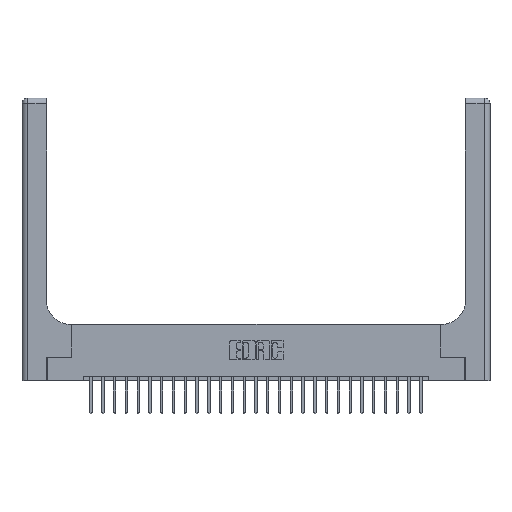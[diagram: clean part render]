
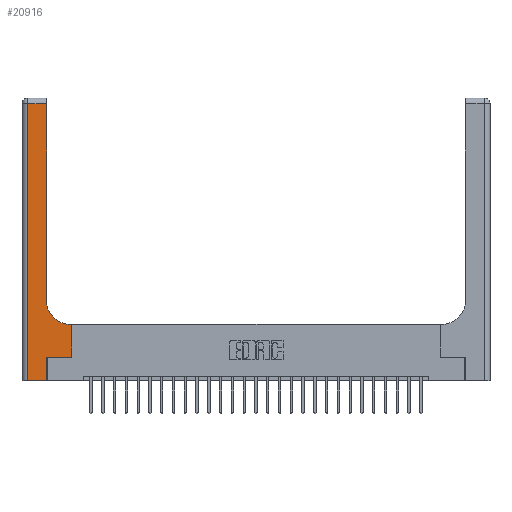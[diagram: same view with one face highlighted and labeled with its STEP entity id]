
A CAD part, top view. The second image highlights one B-rep face of the part: STEP entity #20916.
In plain terms, the highlighted planar face has unit normal (0, 0, 1).
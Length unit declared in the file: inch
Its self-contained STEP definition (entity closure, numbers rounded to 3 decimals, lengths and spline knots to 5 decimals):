
#39 = CARTESIAN_POINT ( 'NONE',  ( 0.26, 2.94, 0.37 ) ) ;
#159 = FACE_OUTER_BOUND ( 'NONE', #4325, .T. ) ;
#354 = AXIS2_PLACEMENT_3D ( 'NONE', #4958, #20908, #21158 ) ;
#686 = EDGE_CURVE ( 'NONE', #1787, #7009, #1585, .T. ) ;
#1585 = LINE ( 'NONE', #11307, #15979 ) ;
#1787 = VERTEX_POINT ( 'NONE', #18577 ) ;
#2803 = LINE ( 'NONE', #23126, #4968 ) ;
#3049 = ORIENTED_EDGE ( 'NONE', *, *, #11460, .T. ) ;
#3132 = DIRECTION ( 'NONE',  ( 1., 0., 0. ) ) ;
#3763 = CARTESIAN_POINT ( 'NONE',  ( 0.265, 0.25, 0.37 ) ) ;
#3944 = LINE ( 'NONE', #15040, #24601 ) ;
#4077 = DIRECTION ( 'NONE',  ( 1., 0., 0. ) ) ;
#4268 = EDGE_CURVE ( 'NONE', #22924, #23371, #23601, .T. ) ;
#4287 = VECTOR ( 'NONE', #4077, 39.37008 ) ;
#4325 = EDGE_LOOP ( 'NONE', ( #24033, #16452, #8283, #21528, #11628, #3049, #9214, #11982, #5911 ) ) ;
#4958 = CARTESIAN_POINT ( 'NONE',  ( 0., 3., 0.37 ) ) ;
#4968 = VECTOR ( 'NONE', #11171, 39.37008 ) ;
#5133 = CARTESIAN_POINT ( 'NONE',  ( 0.265, 0.25, 0.37 ) ) ;
#5168 = CIRCLE ( 'NONE', #20478, 0.25 ) ;
#5269 = LINE ( 'NONE', #14462, #11558 ) ;
#5911 = ORIENTED_EDGE ( 'NONE', *, *, #21114, .T. ) ;
#6788 = DIRECTION ( 'NONE',  ( 0., 1., 0. ) ) ;
#7009 = VERTEX_POINT ( 'NONE', #15015 ) ;
#7729 = VERTEX_POINT ( 'NONE', #3763 ) ;
#8283 = ORIENTED_EDGE ( 'NONE', *, *, #4268, .T. ) ;
#8541 = CARTESIAN_POINT ( 'NONE',  ( 0.265, 0., 0.37 ) ) ;
#8837 = PLANE ( 'NONE',  #354 ) ;
#8862 = DIRECTION ( 'NONE',  ( 0., 1., 0. ) ) ;
#9208 = DIRECTION ( 'NONE',  ( 0., -1., 0. ) ) ;
#9214 = ORIENTED_EDGE ( 'NONE', *, *, #18921, .T. ) ;
#9443 = DIRECTION ( 'NONE',  ( -1., 0., 0. ) ) ;
#9606 = VERTEX_POINT ( 'NONE', #39 ) ;
#10242 = CARTESIAN_POINT ( 'NONE',  ( 0.528, 0.25, 0.37 ) ) ;
#10453 = VECTOR ( 'NONE', #3132, 39.37008 ) ;
#10705 = CARTESIAN_POINT ( 'NONE',  ( 0.26, 0.85, 0.37 ) ) ;
#11039 = CARTESIAN_POINT ( 'NONE',  ( 0.06, 2.94, 0.37 ) ) ;
#11171 = DIRECTION ( 'NONE',  ( 0., 1., 0. ) ) ;
#11202 = DIRECTION ( 'NONE',  ( 1., 0., 0. ) ) ;
#11307 = CARTESIAN_POINT ( 'NONE',  ( 0.26, 0.6, 0.37 ) ) ;
#11460 = EDGE_CURVE ( 'NONE', #7729, #16815, #21092, .T. ) ;
#11558 = VECTOR ( 'NONE', #8862, 39.37008 ) ;
#11628 = ORIENTED_EDGE ( 'NONE', *, *, #12660, .T. ) ;
#11982 = ORIENTED_EDGE ( 'NONE', *, *, #686, .T. ) ;
#12076 = EDGE_CURVE ( 'NONE', #22211, #9606, #2803, .T. ) ;
#12660 = EDGE_CURVE ( 'NONE', #19559, #7729, #5269, .T. ) ;
#13551 = EDGE_CURVE ( 'NONE', #23371, #19559, #14632, .T. ) ;
#14462 = CARTESIAN_POINT ( 'NONE',  ( 0.265, 0., 0.37 ) ) ;
#14498 = EDGE_CURVE ( 'NONE', #9606, #22924, #3944, .T. ) ;
#14632 = LINE ( 'NONE', #23952, #4287 ) ;
#15015 = CARTESIAN_POINT ( 'NONE',  ( 0.51, 0.6, 0.37 ) ) ;
#15040 = CARTESIAN_POINT ( 'NONE',  ( 0., 2.94, 0.37 ) ) ;
#15278 = VECTOR ( 'NONE', #6788, 39.37008 ) ;
#15329 = DIRECTION ( 'NONE',  ( -1., 0., 0. ) ) ;
#15979 = VECTOR ( 'NONE', #15329, 39.37008 ) ;
#16452 = ORIENTED_EDGE ( 'NONE', *, *, #14498, .T. ) ;
#16593 = CARTESIAN_POINT ( 'NONE',  ( 0.528, 0.25, 0.37 ) ) ;
#16815 = VERTEX_POINT ( 'NONE', #10242 ) ;
#17802 = LINE ( 'NONE', #16593, #15278 ) ;
#18577 = CARTESIAN_POINT ( 'NONE',  ( 0.528, 0.6, 0.37 ) ) ;
#18921 = EDGE_CURVE ( 'NONE', #16815, #1787, #17802, .T. ) ;
#19547 = VECTOR ( 'NONE', #9208, 39.37008 ) ;
#19559 = VERTEX_POINT ( 'NONE', #8541 ) ;
#19587 = DIRECTION ( 'NONE',  ( 0., 0., -1. ) ) ;
#20478 = AXIS2_PLACEMENT_3D ( 'NONE', #21573, #19587, #11202 ) ;
#20908 = DIRECTION ( 'NONE',  ( 0., 0., -1. ) ) ;
#20916 = ADVANCED_FACE ( 'NONE', ( #159 ), #8837, .F. ) ;
#21092 = LINE ( 'NONE', #5133, #10453 ) ;
#21114 = EDGE_CURVE ( 'NONE', #7009, #22211, #5168, .T. ) ;
#21158 = DIRECTION ( 'NONE',  ( -1., 0., 0. ) ) ;
#21528 = ORIENTED_EDGE ( 'NONE', *, *, #13551, .T. ) ;
#21573 = CARTESIAN_POINT ( 'NONE',  ( 0.51, 0.85, 0.37 ) ) ;
#22211 = VERTEX_POINT ( 'NONE', #10705 ) ;
#22924 = VERTEX_POINT ( 'NONE', #11039 ) ;
#23126 = CARTESIAN_POINT ( 'NONE',  ( 0.26, 3., 0.37 ) ) ;
#23347 = CARTESIAN_POINT ( 'NONE',  ( 0.06, 3., 0.37 ) ) ;
#23371 = VERTEX_POINT ( 'NONE', #24559 ) ;
#23601 = LINE ( 'NONE', #23347, #19547 ) ;
#23952 = CARTESIAN_POINT ( 'NONE',  ( 0., 0., 0.37 ) ) ;
#24033 = ORIENTED_EDGE ( 'NONE', *, *, #12076, .T. ) ;
#24559 = CARTESIAN_POINT ( 'NONE',  ( 0.06, 0., 0.37 ) ) ;
#24601 = VECTOR ( 'NONE', #9443, 39.37008 ) ;
